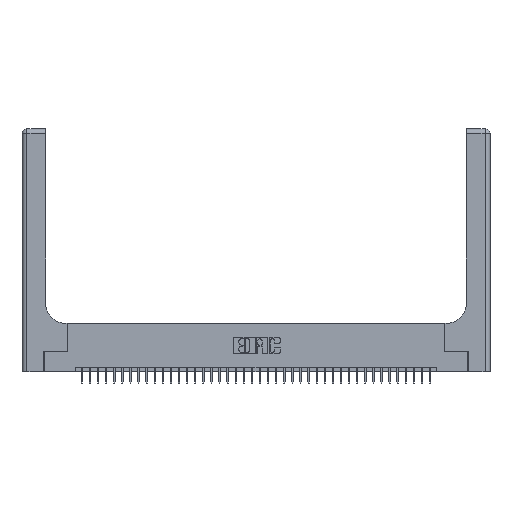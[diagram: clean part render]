
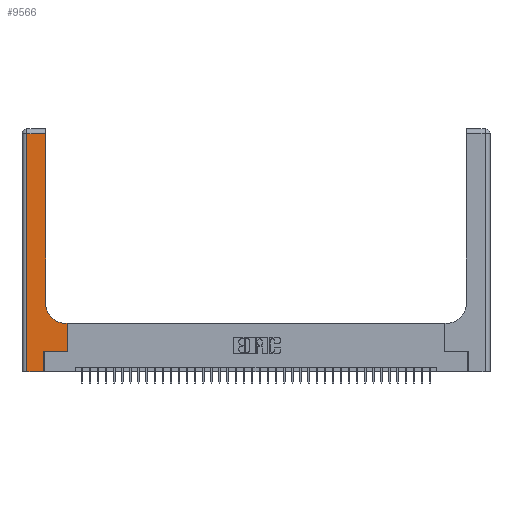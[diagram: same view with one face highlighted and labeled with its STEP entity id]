
A CAD part, top view. The second image highlights one B-rep face of the part: STEP entity #9566.
In plain terms, the highlighted planar face has unit normal (0, 0, 1).
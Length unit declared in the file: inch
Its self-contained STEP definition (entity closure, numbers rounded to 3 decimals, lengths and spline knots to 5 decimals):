
#120 = DIRECTION ( 'NONE',  ( 0., 1., 0. ) ) ;
#181 = LINE ( 'NONE', #30194, #18846 ) ;
#384 = CARTESIAN_POINT ( 'NONE',  ( 0.5415, 0.6, 0.37 ) ) ;
#1358 = ORIENTED_EDGE ( 'NONE', *, *, #13943, .T. ) ;
#1698 = VECTOR ( 'NONE', #36888, 39.37008 ) ;
#1810 = LINE ( 'NONE', #26803, #26060 ) ;
#1858 = CARTESIAN_POINT ( 'NONE',  ( 0.5585, 0.6, 0.37 ) ) ;
#1972 = AXIS2_PLACEMENT_3D ( 'NONE', #12942, #19127, #10138 ) ;
#2278 = VERTEX_POINT ( 'NONE', #39396 ) ;
#3013 = VERTEX_POINT ( 'NONE', #22925 ) ;
#3119 = CARTESIAN_POINT ( 'NONE',  ( 0., 0., 0.37 ) ) ;
#3127 = CARTESIAN_POINT ( 'NONE',  ( 0.269, 0., 0.37 ) ) ;
#3268 = LINE ( 'NONE', #15076, #1698 ) ;
#5797 = DIRECTION ( 'NONE',  ( -1., 0., 0. ) ) ;
#6134 = LINE ( 'NONE', #3119, #8821 ) ;
#6842 = DIRECTION ( 'NONE',  ( 0., 1., 0. ) ) ;
#6936 = FACE_OUTER_BOUND ( 'NONE', #39062, .T. ) ;
#7000 = EDGE_CURVE ( 'NONE', #37030, #23857, #9731, .T. ) ;
#7016 = DIRECTION ( 'NONE',  ( 0., -1., 0. ) ) ;
#8821 = VECTOR ( 'NONE', #12933, 39.37008 ) ;
#8829 = VERTEX_POINT ( 'NONE', #1858 ) ;
#9395 = ORIENTED_EDGE ( 'NONE', *, *, #17420, .T. ) ;
#9566 = ADVANCED_FACE ( 'NONE', ( #6936 ), #22337, .F. ) ;
#9731 = LINE ( 'NONE', #3127, #21020 ) ;
#10138 = DIRECTION ( 'NONE',  ( -1., 0., 0. ) ) ;
#10213 = LINE ( 'NONE', #24821, #21431 ) ;
#10738 = EDGE_CURVE ( 'NONE', #8829, #23484, #1810, .T. ) ;
#11744 = EDGE_CURVE ( 'NONE', #2278, #8829, #28056, .T. ) ;
#11841 = DIRECTION ( 'NONE',  ( 1., 0., 0. ) ) ;
#12253 = CARTESIAN_POINT ( 'NONE',  ( 0.2915, 0.85, 0.37 ) ) ;
#12639 = CIRCLE ( 'NONE', #20285, 0.25 ) ;
#12933 = DIRECTION ( 'NONE',  ( 1., 0., 0. ) ) ;
#12942 = CARTESIAN_POINT ( 'NONE',  ( 0., 3., 0.37 ) ) ;
#13943 = EDGE_CURVE ( 'NONE', #24411, #33682, #181, .T. ) ;
#15076 = CARTESIAN_POINT ( 'NONE',  ( 0., 2.94, 0.37 ) ) ;
#15641 = CARTESIAN_POINT ( 'NONE',  ( 0.5415, 0.85, 0.37 ) ) ;
#17420 = EDGE_CURVE ( 'NONE', #23857, #2278, #35944, .T. ) ;
#17711 = ORIENTED_EDGE ( 'NONE', *, *, #10738, .T. ) ;
#18846 = VECTOR ( 'NONE', #27209, 39.37008 ) ;
#19127 = DIRECTION ( 'NONE',  ( 0., 0., -1. ) ) ;
#20285 = AXIS2_PLACEMENT_3D ( 'NONE', #15641, #39257, #11841 ) ;
#20622 = ORIENTED_EDGE ( 'NONE', *, *, #7000, .T. ) ;
#20721 = CARTESIAN_POINT ( 'NONE',  ( 0.269, 0.25, 0.37 ) ) ;
#21020 = VECTOR ( 'NONE', #120, 39.37008 ) ;
#21431 = VECTOR ( 'NONE', #7016, 39.37008 ) ;
#22337 = PLANE ( 'NONE',  #1972 ) ;
#22788 = CARTESIAN_POINT ( 'NONE',  ( 0.269, 0.25, 0.37 ) ) ;
#22925 = CARTESIAN_POINT ( 'NONE',  ( 0.06, 0., 0.37 ) ) ;
#23117 = EDGE_CURVE ( 'NONE', #23484, #24411, #12639, .T. ) ;
#23484 = VERTEX_POINT ( 'NONE', #384 ) ;
#23857 = VERTEX_POINT ( 'NONE', #22788 ) ;
#24411 = VERTEX_POINT ( 'NONE', #12253 ) ;
#24480 = CARTESIAN_POINT ( 'NONE',  ( 0.269, 0., 0.37 ) ) ;
#24821 = CARTESIAN_POINT ( 'NONE',  ( 0.06, 3., 0.37 ) ) ;
#26060 = VECTOR ( 'NONE', #5797, 39.37008 ) ;
#26803 = CARTESIAN_POINT ( 'NONE',  ( 0.2915, 0.6, 0.37 ) ) ;
#26948 = EDGE_CURVE ( 'NONE', #3013, #37030, #6134, .T. ) ;
#26996 = ORIENTED_EDGE ( 'NONE', *, *, #35596, .T. ) ;
#27209 = DIRECTION ( 'NONE',  ( 0., 1., 0. ) ) ;
#27396 = CARTESIAN_POINT ( 'NONE',  ( 0.06, 2.94, 0.37 ) ) ;
#28056 = LINE ( 'NONE', #34255, #35702 ) ;
#28464 = ORIENTED_EDGE ( 'NONE', *, *, #23117, .T. ) ;
#28908 = ORIENTED_EDGE ( 'NONE', *, *, #26948, .T. ) ;
#30194 = CARTESIAN_POINT ( 'NONE',  ( 0.2915, 3., 0.37 ) ) ;
#31067 = CARTESIAN_POINT ( 'NONE',  ( 0.2915, 2.94, 0.37 ) ) ;
#32219 = ORIENTED_EDGE ( 'NONE', *, *, #11744, .T. ) ;
#32940 = DIRECTION ( 'NONE',  ( 1., 0., 0. ) ) ;
#33682 = VERTEX_POINT ( 'NONE', #31067 ) ;
#34255 = CARTESIAN_POINT ( 'NONE',  ( 0.5585, 0.25, 0.37 ) ) ;
#34339 = EDGE_CURVE ( 'NONE', #37913, #3013, #10213, .T. ) ;
#35596 = EDGE_CURVE ( 'NONE', #33682, #37913, #3268, .T. ) ;
#35702 = VECTOR ( 'NONE', #6842, 39.37008 ) ;
#35944 = LINE ( 'NONE', #20721, #39277 ) ;
#36888 = DIRECTION ( 'NONE',  ( -1., 0., 0. ) ) ;
#37030 = VERTEX_POINT ( 'NONE', #24480 ) ;
#37551 = ORIENTED_EDGE ( 'NONE', *, *, #34339, .T. ) ;
#37913 = VERTEX_POINT ( 'NONE', #27396 ) ;
#39062 = EDGE_LOOP ( 'NONE', ( #1358, #26996, #37551, #28908, #20622, #9395, #32219, #17711, #28464 ) ) ;
#39257 = DIRECTION ( 'NONE',  ( 0., 0., -1. ) ) ;
#39277 = VECTOR ( 'NONE', #32940, 39.37008 ) ;
#39396 = CARTESIAN_POINT ( 'NONE',  ( 0.5585, 0.25, 0.37 ) ) ;
